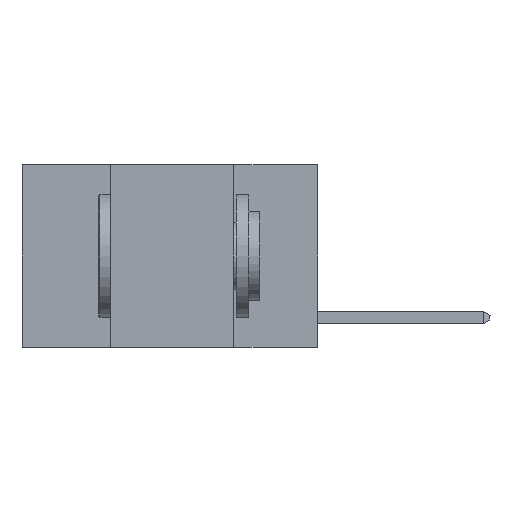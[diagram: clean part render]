
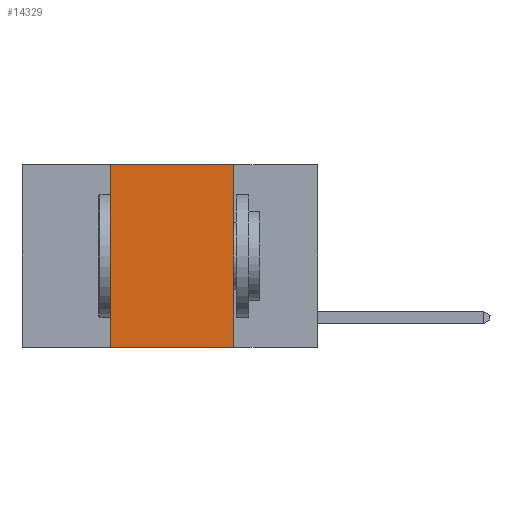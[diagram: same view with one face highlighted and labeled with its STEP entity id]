
A CAD part, left-side view. The second image highlights one B-rep face of the part: STEP entity #14329.
In plain terms, the highlighted planar face has unit normal (-1, 0, 0).
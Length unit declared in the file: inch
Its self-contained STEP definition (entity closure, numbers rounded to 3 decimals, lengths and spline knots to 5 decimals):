
#318 = FACE_OUTER_BOUND ( 'NONE', #11341, .T. ) ;
#589 = CARTESIAN_POINT ( 'NONE',  ( 0., 0.17, 0. ) ) ;
#647 = ORIENTED_EDGE ( 'NONE', *, *, #1652, .F. ) ;
#1456 = LINE ( 'NONE', #13057, #17526 ) ;
#1652 = EDGE_CURVE ( 'NONE', #16998, #5727, #1456, .T. ) ;
#1849 = DIRECTION ( 'NONE',  ( 1., 0., 0. ) ) ;
#2161 = CARTESIAN_POINT ( 'NONE',  ( 0., 0.6, -0.37 ) ) ;
#2248 = LINE ( 'NONE', #7290, #7459 ) ;
#2722 = EDGE_CURVE ( 'NONE', #16998, #9118, #14205, .T. ) ;
#2997 = LINE ( 'NONE', #589, #17213 ) ;
#3704 = CARTESIAN_POINT ( 'NONE',  ( 0., 0.17, 0. ) ) ;
#4175 = AXIS2_PLACEMENT_3D ( 'NONE', #12592, #1849, #15134 ) ;
#4458 = VERTEX_POINT ( 'NONE', #3704 ) ;
#5727 = VERTEX_POINT ( 'NONE', #7517 ) ;
#7290 = CARTESIAN_POINT ( 'NONE',  ( 0., 0.6, 0. ) ) ;
#7453 = ORIENTED_EDGE ( 'NONE', *, *, #9325, .F. ) ;
#7459 = VECTOR ( 'NONE', #14130, 39.37008 ) ;
#7517 = CARTESIAN_POINT ( 'NONE',  ( 0., 0.42, 0. ) ) ;
#7560 = ORIENTED_EDGE ( 'NONE', *, *, #12520, .F. ) ;
#9118 = VERTEX_POINT ( 'NONE', #15006 ) ;
#9325 = EDGE_CURVE ( 'NONE', #5727, #4458, #2248, .T. ) ;
#9635 = VECTOR ( 'NONE', #11580, 39.37008 ) ;
#9923 = PLANE ( 'NONE',  #4175 ) ;
#9927 = DIRECTION ( 'NONE',  ( 0., 0., -1. ) ) ;
#10475 = CARTESIAN_POINT ( 'NONE',  ( 0., 0.42, -0.37 ) ) ;
#11341 = EDGE_LOOP ( 'NONE', ( #7560, #7453, #647, #13310 ) ) ;
#11580 = DIRECTION ( 'NONE',  ( 0., -1., 0. ) ) ;
#12520 = EDGE_CURVE ( 'NONE', #4458, #9118, #2997, .T. ) ;
#12592 = CARTESIAN_POINT ( 'NONE',  ( 0., 0.6, 0. ) ) ;
#13057 = CARTESIAN_POINT ( 'NONE',  ( 0., 0.42, 0. ) ) ;
#13310 = ORIENTED_EDGE ( 'NONE', *, *, #2722, .T. ) ;
#14130 = DIRECTION ( 'NONE',  ( 0., -1., 0. ) ) ;
#14205 = LINE ( 'NONE', #2161, #9635 ) ;
#14329 = ADVANCED_FACE ( 'NONE', ( #318 ), #9923, .F. ) ;
#15006 = CARTESIAN_POINT ( 'NONE',  ( 0., 0.17, -0.37 ) ) ;
#15134 = DIRECTION ( 'NONE',  ( 0., 0., -1. ) ) ;
#16998 = VERTEX_POINT ( 'NONE', #10475 ) ;
#17213 = VECTOR ( 'NONE', #9927, 39.37008 ) ;
#17515 = DIRECTION ( 'NONE',  ( 0., 0., 1. ) ) ;
#17526 = VECTOR ( 'NONE', #17515, 39.37008 ) ;
